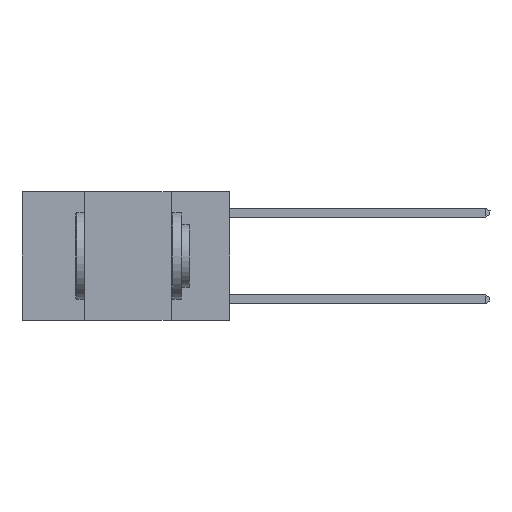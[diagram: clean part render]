
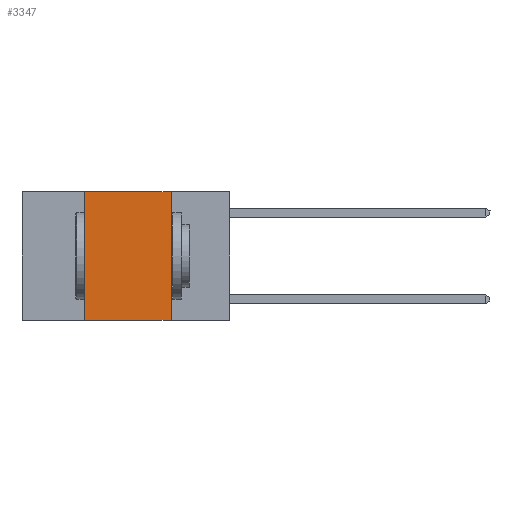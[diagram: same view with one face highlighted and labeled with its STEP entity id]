
A CAD part, left-side view. The second image highlights one B-rep face of the part: STEP entity #3347.
In plain terms, the highlighted planar face has unit normal (-1, 0, 0).
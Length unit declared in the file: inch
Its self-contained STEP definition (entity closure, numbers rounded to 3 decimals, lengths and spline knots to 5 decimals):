
#419 = AXIS2_PLACEMENT_3D ( 'NONE', #5797, #5526, #5468 ) ;
#1254 = VECTOR ( 'NONE', #13609, 39.37008 ) ;
#1327 = DIRECTION ( 'NONE',  ( 0., -1., 0. ) ) ;
#1538 = VERTEX_POINT ( 'NONE', #3497 ) ;
#2629 = CARTESIAN_POINT ( 'NONE',  ( 0., 0.42, -0.37 ) ) ;
#2945 = VERTEX_POINT ( 'NONE', #13662 ) ;
#3347 = ADVANCED_FACE ( 'NONE', ( #4863 ), #5583, .F. ) ;
#3497 = CARTESIAN_POINT ( 'NONE',  ( 0., 0.17, 0. ) ) ;
#3696 = CARTESIAN_POINT ( 'NONE',  ( 0., 0.42, 0. ) ) ;
#3859 = CARTESIAN_POINT ( 'NONE',  ( 0., 0.6, 0. ) ) ;
#4292 = LINE ( 'NONE', #4749, #1254 ) ;
#4657 = VECTOR ( 'NONE', #1327, 39.37008 ) ;
#4749 = CARTESIAN_POINT ( 'NONE',  ( 0., 0.6, -0.37 ) ) ;
#4863 = FACE_OUTER_BOUND ( 'NONE', #15701, .T. ) ;
#4999 = VECTOR ( 'NONE', #10599, 39.37008 ) ;
#5468 = DIRECTION ( 'NONE',  ( 0., 0., -1. ) ) ;
#5522 = EDGE_CURVE ( 'NONE', #15445, #10308, #4292, .T. ) ;
#5526 = DIRECTION ( 'NONE',  ( 1., 0., 0. ) ) ;
#5583 = PLANE ( 'NONE',  #419 ) ;
#5797 = CARTESIAN_POINT ( 'NONE',  ( 0., 0.6, 0. ) ) ;
#5841 = VECTOR ( 'NONE', #13851, 39.37008 ) ;
#6370 = EDGE_CURVE ( 'NONE', #15445, #2945, #15859, .T. ) ;
#6465 = EDGE_CURVE ( 'NONE', #2945, #1538, #15107, .T. ) ;
#6780 = CARTESIAN_POINT ( 'NONE',  ( 0., 0.17, 0. ) ) ;
#8266 = EDGE_CURVE ( 'NONE', #1538, #10308, #8301, .T. ) ;
#8301 = LINE ( 'NONE', #6780, #4999 ) ;
#9363 = ORIENTED_EDGE ( 'NONE', *, *, #8266, .F. ) ;
#10167 = CARTESIAN_POINT ( 'NONE',  ( 0., 0.17, -0.37 ) ) ;
#10308 = VERTEX_POINT ( 'NONE', #10167 ) ;
#10599 = DIRECTION ( 'NONE',  ( 0., 0., -1. ) ) ;
#12095 = ORIENTED_EDGE ( 'NONE', *, *, #6465, .F. ) ;
#12878 = ORIENTED_EDGE ( 'NONE', *, *, #5522, .T. ) ;
#12900 = ORIENTED_EDGE ( 'NONE', *, *, #6370, .F. ) ;
#13609 = DIRECTION ( 'NONE',  ( 0., -1., 0. ) ) ;
#13662 = CARTESIAN_POINT ( 'NONE',  ( 0., 0.42, 0. ) ) ;
#13851 = DIRECTION ( 'NONE',  ( 0., 0., 1. ) ) ;
#15107 = LINE ( 'NONE', #3859, #4657 ) ;
#15445 = VERTEX_POINT ( 'NONE', #2629 ) ;
#15701 = EDGE_LOOP ( 'NONE', ( #9363, #12095, #12900, #12878 ) ) ;
#15859 = LINE ( 'NONE', #3696, #5841 ) ;
